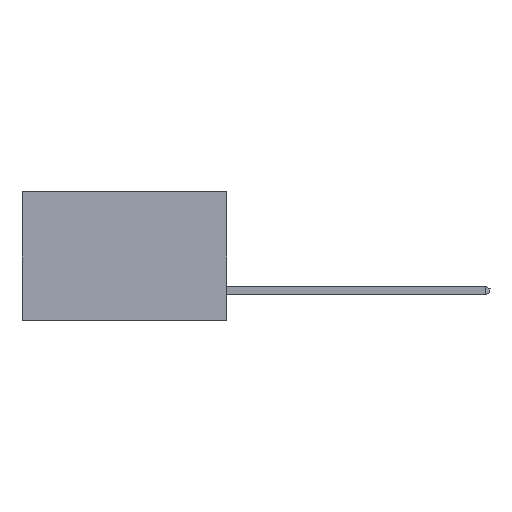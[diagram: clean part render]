
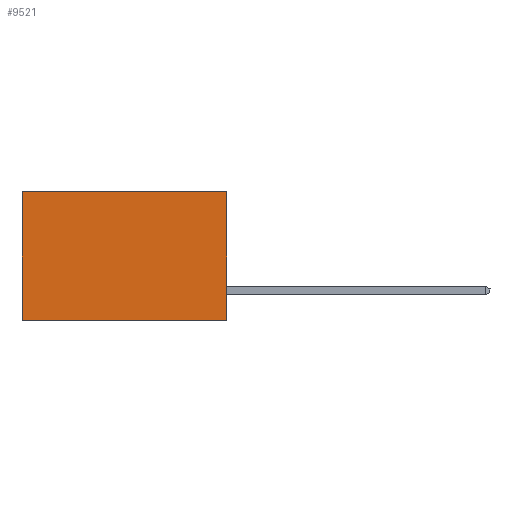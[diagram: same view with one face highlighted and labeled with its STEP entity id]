
A CAD part, left-side view. The second image highlights one B-rep face of the part: STEP entity #9521.
In plain terms, the highlighted planar face has unit normal (-1, 0, 0).
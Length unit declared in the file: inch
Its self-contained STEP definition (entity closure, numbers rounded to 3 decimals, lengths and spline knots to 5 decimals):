
#614 = AXIS2_PLACEMENT_3D ( 'NONE', #17279, #13033, #4114 ) ;
#1028 = DIRECTION ( 'NONE',  ( 0., 1., 0. ) ) ;
#1400 = EDGE_LOOP ( 'NONE', ( #18242, #7039, #18677, #15320 ) ) ;
#2604 = PLANE ( 'NONE',  #614 ) ;
#3128 = VERTEX_POINT ( 'NONE', #5037 ) ;
#3743 = CARTESIAN_POINT ( 'NONE',  ( 0.277, 0., -0.37 ) ) ;
#3754 = VERTEX_POINT ( 'NONE', #11859 ) ;
#4114 = DIRECTION ( 'NONE',  ( 0., 0., -1. ) ) ;
#4941 = VECTOR ( 'NONE', #9806, 39.37008 ) ;
#4981 = VERTEX_POINT ( 'NONE', #8334 ) ;
#5037 = CARTESIAN_POINT ( 'NONE',  ( 0.277, 0., 0. ) ) ;
#5839 = FACE_OUTER_BOUND ( 'NONE', #1400, .T. ) ;
#6431 = CARTESIAN_POINT ( 'NONE',  ( 0.277, 0.59, -0.37 ) ) ;
#7039 = ORIENTED_EDGE ( 'NONE', *, *, #8729, .F. ) ;
#7979 = VECTOR ( 'NONE', #1028, 39.37008 ) ;
#8334 = CARTESIAN_POINT ( 'NONE',  ( 0.277, 0., -0.37 ) ) ;
#8674 = EDGE_CURVE ( 'NONE', #3754, #10580, #16674, .T. ) ;
#8729 = EDGE_CURVE ( 'NONE', #4981, #10580, #15775, .T. ) ;
#9333 = LINE ( 'NONE', #13285, #16620 ) ;
#9521 = ADVANCED_FACE ( 'NONE', ( #5839 ), #2604, .F. ) ;
#9806 = DIRECTION ( 'NONE',  ( 0., 0., -1. ) ) ;
#10580 = VERTEX_POINT ( 'NONE', #6431 ) ;
#11474 = CARTESIAN_POINT ( 'NONE',  ( 0.277, 0., -0.37 ) ) ;
#11859 = CARTESIAN_POINT ( 'NONE',  ( 0.277, 0.59, 0. ) ) ;
#13033 = DIRECTION ( 'NONE',  ( 1., 0., 0. ) ) ;
#13285 = CARTESIAN_POINT ( 'NONE',  ( 0.277, 0., 0. ) ) ;
#14103 = DIRECTION ( 'NONE',  ( 0., 0., -1. ) ) ;
#14702 = DIRECTION ( 'NONE',  ( 0., 1., 0. ) ) ;
#14842 = LINE ( 'NONE', #3743, #18667 ) ;
#15014 = EDGE_CURVE ( 'NONE', #3128, #4981, #14842, .T. ) ;
#15320 = ORIENTED_EDGE ( 'NONE', *, *, #15324, .T. ) ;
#15324 = EDGE_CURVE ( 'NONE', #3128, #3754, #9333, .T. ) ;
#15775 = LINE ( 'NONE', #11474, #7979 ) ;
#16620 = VECTOR ( 'NONE', #14702, 39.37008 ) ;
#16674 = LINE ( 'NONE', #17052, #4941 ) ;
#17052 = CARTESIAN_POINT ( 'NONE',  ( 0.277, 0.59, -0.37 ) ) ;
#17279 = CARTESIAN_POINT ( 'NONE',  ( 0.277, 0., -0.37 ) ) ;
#18242 = ORIENTED_EDGE ( 'NONE', *, *, #8674, .T. ) ;
#18667 = VECTOR ( 'NONE', #14103, 39.37008 ) ;
#18677 = ORIENTED_EDGE ( 'NONE', *, *, #15014, .F. ) ;
